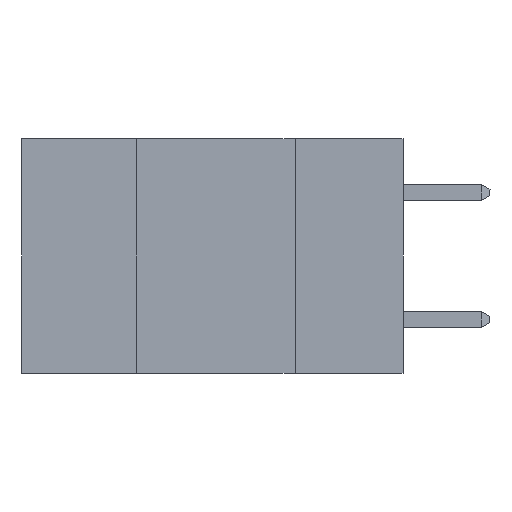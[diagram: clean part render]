
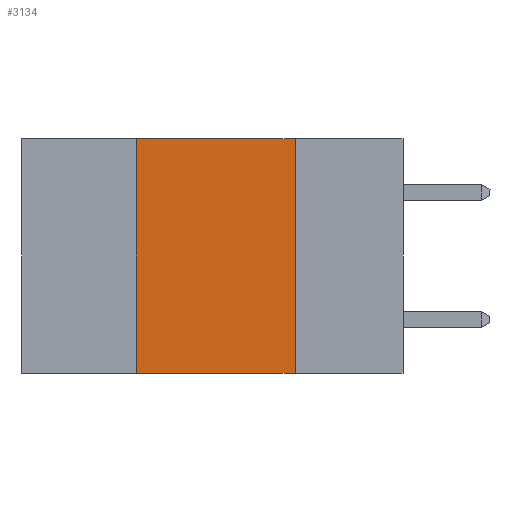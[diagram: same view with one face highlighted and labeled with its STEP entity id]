
A CAD part, left-side view. The second image highlights one B-rep face of the part: STEP entity #3134.
In plain terms, the highlighted planar face has unit normal (-1, 0, 0).
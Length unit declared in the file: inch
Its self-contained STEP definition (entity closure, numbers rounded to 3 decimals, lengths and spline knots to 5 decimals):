
#282 = DIRECTION ( 'NONE',  ( 1., 0., 0. ) ) ;
#918 = VERTEX_POINT ( 'NONE', #9208 ) ;
#1129 = CARTESIAN_POINT ( 'NONE',  ( 0., 0.42, -0.37 ) ) ;
#1159 = DIRECTION ( 'NONE',  ( 0., -1., 0. ) ) ;
#1467 = DIRECTION ( 'NONE',  ( 0., 0., -1. ) ) ;
#1806 = FACE_OUTER_BOUND ( 'NONE', #9918, .T. ) ;
#1946 = CARTESIAN_POINT ( 'NONE',  ( 0., 0.42, 0. ) ) ;
#2387 = CARTESIAN_POINT ( 'NONE',  ( 0., 0.17, 0. ) ) ;
#2501 = LINE ( 'NONE', #2387, #6742 ) ;
#2862 = DIRECTION ( 'NONE',  ( 0., 0., 1. ) ) ;
#3003 = VECTOR ( 'NONE', #6236, 39.37008 ) ;
#3025 = CARTESIAN_POINT ( 'NONE',  ( 0., 0.6, 0. ) ) ;
#3134 = ADVANCED_FACE ( 'NONE', ( #1806 ), #4177, .F. ) ;
#3707 = VERTEX_POINT ( 'NONE', #4023 ) ;
#3735 = ORIENTED_EDGE ( 'NONE', *, *, #3799, .F. ) ;
#3799 = EDGE_CURVE ( 'NONE', #918, #3707, #2501, .T. ) ;
#4023 = CARTESIAN_POINT ( 'NONE',  ( 0., 0.17, -0.37 ) ) ;
#4177 = PLANE ( 'NONE',  #7449 ) ;
#4317 = CARTESIAN_POINT ( 'NONE',  ( 0., 0.42, 0. ) ) ;
#5222 = LINE ( 'NONE', #5417, #3003 ) ;
#5417 = CARTESIAN_POINT ( 'NONE',  ( 0., 0.6, -0.37 ) ) ;
#5543 = VERTEX_POINT ( 'NONE', #4317 ) ;
#5581 = LINE ( 'NONE', #9594, #9687 ) ;
#6236 = DIRECTION ( 'NONE',  ( 0., -1., 0. ) ) ;
#6614 = VERTEX_POINT ( 'NONE', #1129 ) ;
#6742 = VECTOR ( 'NONE', #1467, 39.37008 ) ;
#6900 = ORIENTED_EDGE ( 'NONE', *, *, #7362, .T. ) ;
#7069 = VECTOR ( 'NONE', #2862, 39.37008 ) ;
#7318 = LINE ( 'NONE', #1946, #7069 ) ;
#7362 = EDGE_CURVE ( 'NONE', #6614, #3707, #5222, .T. ) ;
#7449 = AXIS2_PLACEMENT_3D ( 'NONE', #3025, #282, #7787 ) ;
#7787 = DIRECTION ( 'NONE',  ( 0., 0., -1. ) ) ;
#7902 = EDGE_CURVE ( 'NONE', #6614, #5543, #7318, .T. ) ;
#7951 = ORIENTED_EDGE ( 'NONE', *, *, #10720, .F. ) ;
#8072 = ORIENTED_EDGE ( 'NONE', *, *, #7902, .F. ) ;
#9208 = CARTESIAN_POINT ( 'NONE',  ( 0., 0.17, 0. ) ) ;
#9594 = CARTESIAN_POINT ( 'NONE',  ( 0., 0.6, 0. ) ) ;
#9687 = VECTOR ( 'NONE', #1159, 39.37008 ) ;
#9918 = EDGE_LOOP ( 'NONE', ( #3735, #7951, #8072, #6900 ) ) ;
#10720 = EDGE_CURVE ( 'NONE', #5543, #918, #5581, .T. ) ;
